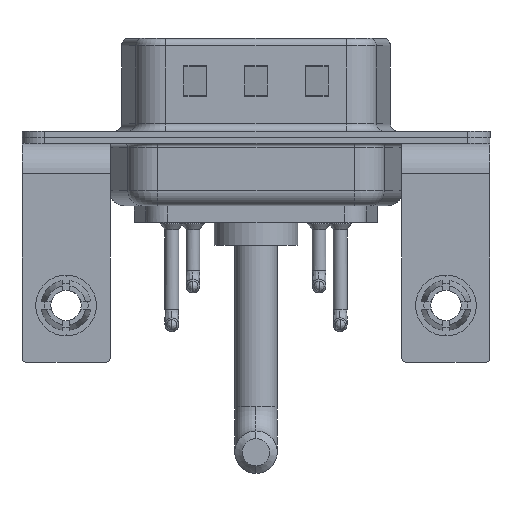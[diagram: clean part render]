
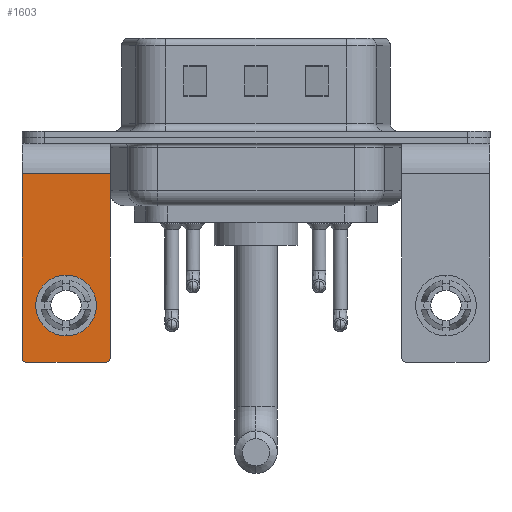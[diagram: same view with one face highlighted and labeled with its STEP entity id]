
A CAD part, front view. The second image highlights one B-rep face of the part: STEP entity #1603.
In plain terms, the highlighted planar face has unit normal (0, -1, 0).
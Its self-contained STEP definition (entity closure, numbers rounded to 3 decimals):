
#114 = CARTESIAN_POINT ( 'NONE',  ( 2.9, -6.25, -2.4 ) ) ;
#725 = LINE ( 'NONE', #932, #15751 ) ;
#932 = CARTESIAN_POINT ( 'NONE',  ( 2.9, -6.25, -2.4 ) ) ;
#1109 = DIRECTION ( 'NONE',  ( 0., -1., 0. ) ) ;
#1603 = ADVANCED_FACE ( 'NONE', ( #7807, #19874 ), #6472, .F. ) ;
#1896 = DIRECTION ( 'NONE',  ( -1., 0., 0. ) ) ;
#2169 = AXIS2_PLACEMENT_3D ( 'NONE', #21563, #1109, #4848 ) ;
#2218 = VECTOR ( 'NONE', #10960, 1000. ) ;
#2511 = VERTEX_POINT ( 'NONE', #17369 ) ;
#2657 = CIRCLE ( 'NONE', #13987, 2. ) ;
#4014 = EDGE_CURVE ( 'NONE', #20835, #20046, #17813, .T. ) ;
#4262 = AXIS2_PLACEMENT_3D ( 'NONE', #20651, #15635, #10887 ) ;
#4407 = EDGE_CURVE ( 'NONE', #2511, #7191, #20564, .T. ) ;
#4676 = VERTEX_POINT ( 'NONE', #7255 ) ;
#4848 = DIRECTION ( 'NONE',  ( 0., 0., 1. ) ) ;
#4961 = VECTOR ( 'NONE', #1896, 1000. ) ;
#5568 = CARTESIAN_POINT ( 'NONE',  ( 0., -6.25, -11.07 ) ) ;
#5760 = EDGE_CURVE ( 'NONE', #19471, #5967, #725, .T. ) ;
#5967 = VERTEX_POINT ( 'NONE', #9857 ) ;
#6002 = LINE ( 'NONE', #17675, #2218 ) ;
#6472 = PLANE ( 'NONE',  #14441 ) ;
#6562 = AXIS2_PLACEMENT_3D ( 'NONE', #14924, #7959, #11287 ) ;
#7191 = VERTEX_POINT ( 'NONE', #12642 ) ;
#7255 = CARTESIAN_POINT ( 'NONE',  ( 2.65, -6.25, -14.8 ) ) ;
#7807 = FACE_BOUND ( 'NONE', #9603, .T. ) ;
#7959 = DIRECTION ( 'NONE',  ( 0., 1., 0. ) ) ;
#8201 = CARTESIAN_POINT ( 'NONE',  ( -2.9, -6.25, -2.4 ) ) ;
#8377 = EDGE_CURVE ( 'NONE', #17084, #2511, #16089, .T. ) ;
#8526 = CARTESIAN_POINT ( 'NONE',  ( 2.9, -6.25, -14.8 ) ) ;
#9603 = EDGE_LOOP ( 'NONE', ( #20182, #16653 ) ) ;
#9663 = EDGE_LOOP ( 'NONE', ( #10885, #15379, #19661, #20780, #14800, #19360 ) ) ;
#9810 = VECTOR ( 'NONE', #12462, 1000. ) ;
#9857 = CARTESIAN_POINT ( 'NONE',  ( 2.9, -6.25, -14.55 ) ) ;
#10129 = EDGE_CURVE ( 'NONE', #4676, #5967, #10234, .T. ) ;
#10234 = CIRCLE ( 'NONE', #4262, 0.25 ) ;
#10885 = ORIENTED_EDGE ( 'NONE', *, *, #8377, .T. ) ;
#10887 = DIRECTION ( 'NONE',  ( 0., 0., 1. ) ) ;
#10960 = DIRECTION ( 'NONE',  ( -1., 0., 0. ) ) ;
#11287 = DIRECTION ( 'NONE',  ( 0., 0., 1. ) ) ;
#12462 = DIRECTION ( 'NONE',  ( 0., 0., -1. ) ) ;
#12485 = EDGE_CURVE ( 'NONE', #20046, #20835, #2657, .T. ) ;
#12642 = CARTESIAN_POINT ( 'NONE',  ( -2.65, -6.25, -14.8 ) ) ;
#12777 = CARTESIAN_POINT ( 'NONE',  ( 0., -6.25, -13.07 ) ) ;
#13314 = CARTESIAN_POINT ( 'NONE',  ( 2.9, -6.25, -2.4 ) ) ;
#13861 = DIRECTION ( 'NONE',  ( 0., 0., 1. ) ) ;
#13987 = AXIS2_PLACEMENT_3D ( 'NONE', #5568, #17027, #13861 ) ;
#14072 = DIRECTION ( 'NONE',  ( 0., 0., -1. ) ) ;
#14327 = CARTESIAN_POINT ( 'NONE',  ( -2.9, -6.25, -2.4 ) ) ;
#14441 = AXIS2_PLACEMENT_3D ( 'NONE', #13314, #19674, #18364 ) ;
#14800 = ORIENTED_EDGE ( 'NONE', *, *, #5760, .F. ) ;
#14924 = CARTESIAN_POINT ( 'NONE',  ( 0., -6.25, -11.07 ) ) ;
#15379 = ORIENTED_EDGE ( 'NONE', *, *, #4407, .T. ) ;
#15635 = DIRECTION ( 'NONE',  ( 0., -1., 0. ) ) ;
#15751 = VECTOR ( 'NONE', #14072, 1000. ) ;
#16089 = LINE ( 'NONE', #14327, #9810 ) ;
#16133 = CARTESIAN_POINT ( 'NONE',  ( 0., -6.25, -9.07 ) ) ;
#16653 = ORIENTED_EDGE ( 'NONE', *, *, #12485, .T. ) ;
#16997 = LINE ( 'NONE', #8526, #4961 ) ;
#17027 = DIRECTION ( 'NONE',  ( 0., 1., 0. ) ) ;
#17046 = EDGE_CURVE ( 'NONE', #4676, #7191, #16997, .T. ) ;
#17084 = VERTEX_POINT ( 'NONE', #8201 ) ;
#17369 = CARTESIAN_POINT ( 'NONE',  ( -2.9, -6.25, -14.55 ) ) ;
#17675 = CARTESIAN_POINT ( 'NONE',  ( 2.9, -6.25, -2.4 ) ) ;
#17813 = CIRCLE ( 'NONE', #6562, 2. ) ;
#18364 = DIRECTION ( 'NONE',  ( 0., 0., 1. ) ) ;
#19360 = ORIENTED_EDGE ( 'NONE', *, *, #21213, .T. ) ;
#19471 = VERTEX_POINT ( 'NONE', #114 ) ;
#19661 = ORIENTED_EDGE ( 'NONE', *, *, #17046, .F. ) ;
#19674 = DIRECTION ( 'NONE',  ( 0., 1., 0. ) ) ;
#19874 = FACE_OUTER_BOUND ( 'NONE', #9663, .T. ) ;
#20046 = VERTEX_POINT ( 'NONE', #16133 ) ;
#20182 = ORIENTED_EDGE ( 'NONE', *, *, #4014, .T. ) ;
#20564 = CIRCLE ( 'NONE', #2169, 0.25 ) ;
#20651 = CARTESIAN_POINT ( 'NONE',  ( 2.65, -6.25, -14.55 ) ) ;
#20780 = ORIENTED_EDGE ( 'NONE', *, *, #10129, .T. ) ;
#20835 = VERTEX_POINT ( 'NONE', #12777 ) ;
#21213 = EDGE_CURVE ( 'NONE', #19471, #17084, #6002, .T. ) ;
#21563 = CARTESIAN_POINT ( 'NONE',  ( -2.65, -6.25, -14.55 ) ) ;
